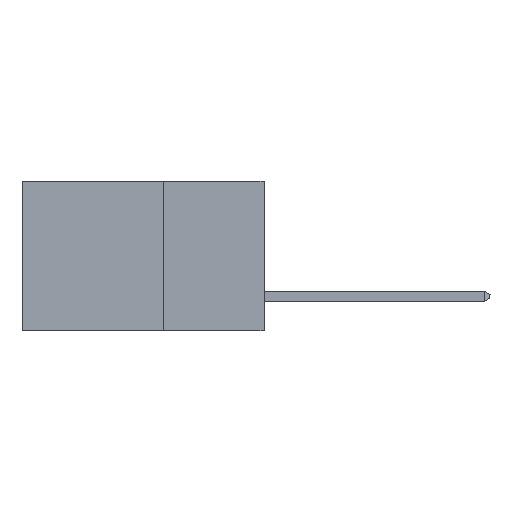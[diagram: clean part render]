
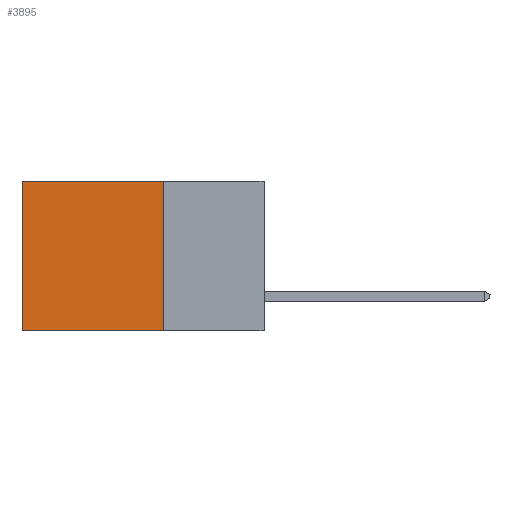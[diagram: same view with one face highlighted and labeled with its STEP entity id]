
A CAD part, left-side view. The second image highlights one B-rep face of the part: STEP entity #3895.
In plain terms, the highlighted planar face has unit normal (-1, 0, 0).
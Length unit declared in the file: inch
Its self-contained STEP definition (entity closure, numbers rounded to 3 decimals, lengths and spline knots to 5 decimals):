
#249 = CARTESIAN_POINT ( 'NONE',  ( 0.298, 0.25, -0.37 ) ) ;
#786 = DIRECTION ( 'NONE',  ( 0., 0., -1. ) ) ;
#1105 = LINE ( 'NONE', #13844, #4895 ) ;
#1986 = EDGE_CURVE ( 'NONE', #16633, #20024, #3152, .T. ) ;
#2092 = FACE_OUTER_BOUND ( 'NONE', #3052, .T. ) ;
#2247 = ORIENTED_EDGE ( 'NONE', *, *, #12027, .F. ) ;
#2843 = EDGE_CURVE ( 'NONE', #20024, #16272, #1105, .T. ) ;
#3052 = EDGE_LOOP ( 'NONE', ( #17879, #2247, #15794, #8954 ) ) ;
#3152 = LINE ( 'NONE', #6491, #5187 ) ;
#3895 = ADVANCED_FACE ( 'NONE', ( #2092 ), #19841, .F. ) ;
#4158 = VECTOR ( 'NONE', #8526, 39.37008 ) ;
#4895 = VECTOR ( 'NONE', #20304, 39.37008 ) ;
#5187 = VECTOR ( 'NONE', #9865, 39.37008 ) ;
#6491 = CARTESIAN_POINT ( 'NONE',  ( 0.298, 0.25, 0. ) ) ;
#8338 = VECTOR ( 'NONE', #18872, 39.37008 ) ;
#8526 = DIRECTION ( 'NONE',  ( 0., 1., 0. ) ) ;
#8670 = CARTESIAN_POINT ( 'NONE',  ( 0.298, 0.25, -0.37 ) ) ;
#8671 = CARTESIAN_POINT ( 'NONE',  ( 0.298, 0.25, 0. ) ) ;
#8954 = ORIENTED_EDGE ( 'NONE', *, *, #1986, .T. ) ;
#8968 = LINE ( 'NONE', #249, #4158 ) ;
#9425 = CARTESIAN_POINT ( 'NONE',  ( 0.298, 0.6, -0.37 ) ) ;
#9865 = DIRECTION ( 'NONE',  ( 0., 1., 0. ) ) ;
#12027 = EDGE_CURVE ( 'NONE', #12212, #16272, #8968, .T. ) ;
#12212 = VERTEX_POINT ( 'NONE', #8670 ) ;
#13158 = CARTESIAN_POINT ( 'NONE',  ( 0.298, 0.6, 0. ) ) ;
#13593 = DIRECTION ( 'NONE',  ( 1., 0., 0. ) ) ;
#13844 = CARTESIAN_POINT ( 'NONE',  ( 0.298, 0.6, 0. ) ) ;
#15794 = ORIENTED_EDGE ( 'NONE', *, *, #19912, .F. ) ;
#15826 = LINE ( 'NONE', #18733, #8338 ) ;
#16272 = VERTEX_POINT ( 'NONE', #9425 ) ;
#16633 = VERTEX_POINT ( 'NONE', #19520 ) ;
#17879 = ORIENTED_EDGE ( 'NONE', *, *, #2843, .T. ) ;
#18733 = CARTESIAN_POINT ( 'NONE',  ( 0.298, 0.25, 0. ) ) ;
#18872 = DIRECTION ( 'NONE',  ( 0., 0., -1. ) ) ;
#19457 = AXIS2_PLACEMENT_3D ( 'NONE', #8671, #13593, #786 ) ;
#19520 = CARTESIAN_POINT ( 'NONE',  ( 0.298, 0.25, 0. ) ) ;
#19841 = PLANE ( 'NONE',  #19457 ) ;
#19912 = EDGE_CURVE ( 'NONE', #16633, #12212, #15826, .T. ) ;
#20024 = VERTEX_POINT ( 'NONE', #13158 ) ;
#20304 = DIRECTION ( 'NONE',  ( 0., 0., -1. ) ) ;
